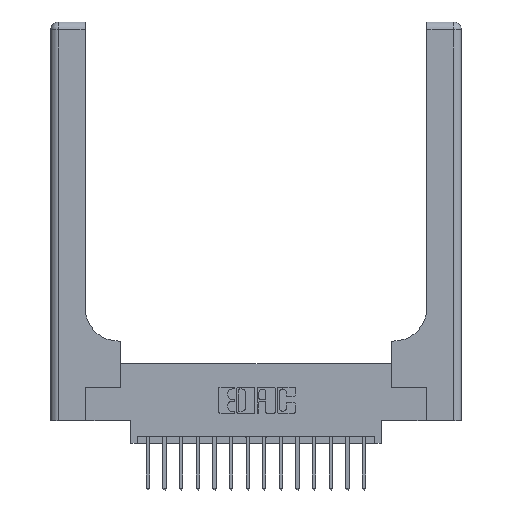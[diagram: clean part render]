
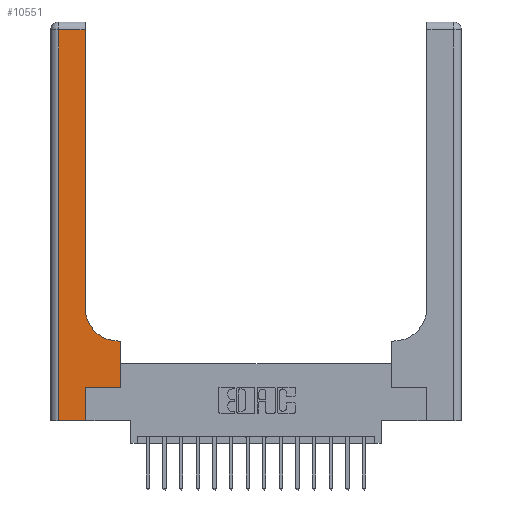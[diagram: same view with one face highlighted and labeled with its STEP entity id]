
A CAD part, top view. The second image highlights one B-rep face of the part: STEP entity #10551.
In plain terms, the highlighted planar face has unit normal (0, 0, 1).
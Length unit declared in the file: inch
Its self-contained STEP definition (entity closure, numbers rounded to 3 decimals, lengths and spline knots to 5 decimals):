
#180 = FACE_OUTER_BOUND ( 'NONE', #14261, .T. ) ;
#314 = LINE ( 'NONE', #7513, #13786 ) ;
#416 = DIRECTION ( 'NONE',  ( 0., 1., 0. ) ) ;
#673 = CARTESIAN_POINT ( 'NONE',  ( 0.26, 0.6, 0.37 ) ) ;
#781 = ORIENTED_EDGE ( 'NONE', *, *, #9626, .T. ) ;
#1243 = CARTESIAN_POINT ( 'NONE',  ( 0.265, 0., 0.37 ) ) ;
#1295 = VECTOR ( 'NONE', #16761, 39.37008 ) ;
#1492 = CARTESIAN_POINT ( 'NONE',  ( 0., 0., 0.37 ) ) ;
#2117 = LINE ( 'NONE', #7989, #9222 ) ;
#2170 = ORIENTED_EDGE ( 'NONE', *, *, #17997, .T. ) ;
#2189 = ORIENTED_EDGE ( 'NONE', *, *, #5326, .T. ) ;
#2384 = CARTESIAN_POINT ( 'NONE',  ( 0.26, 3., 0.37 ) ) ;
#2570 = LINE ( 'NONE', #18563, #8557 ) ;
#2741 = DIRECTION ( 'NONE',  ( 0., 1., 0. ) ) ;
#2985 = PLANE ( 'NONE',  #10521 ) ;
#3191 = VERTEX_POINT ( 'NONE', #1243 ) ;
#3690 = VERTEX_POINT ( 'NONE', #8817 ) ;
#3984 = ORIENTED_EDGE ( 'NONE', *, *, #6276, .T. ) ;
#4375 = VERTEX_POINT ( 'NONE', #17189 ) ;
#4446 = LINE ( 'NONE', #11925, #5252 ) ;
#4491 = CARTESIAN_POINT ( 'NONE',  ( 0.51, 0.6, 0.37 ) ) ;
#5035 = LINE ( 'NONE', #2384, #12600 ) ;
#5252 = VECTOR ( 'NONE', #5945, 39.37008 ) ;
#5265 = EDGE_CURVE ( 'NONE', #6155, #10819, #5832, .T. ) ;
#5299 = EDGE_CURVE ( 'NONE', #3690, #15250, #4446, .T. ) ;
#5326 = EDGE_CURVE ( 'NONE', #4375, #3191, #13040, .T. ) ;
#5688 = CARTESIAN_POINT ( 'NONE',  ( 0.26, 2.94, 0.37 ) ) ;
#5832 = CIRCLE ( 'NONE', #8265, 0.25 ) ;
#5945 = DIRECTION ( 'NONE',  ( 1., 0., 0. ) ) ;
#6155 = VERTEX_POINT ( 'NONE', #4491 ) ;
#6276 = EDGE_CURVE ( 'NONE', #15250, #17471, #2117, .T. ) ;
#6293 = CARTESIAN_POINT ( 'NONE',  ( 0.528, 0.6, 0.37 ) ) ;
#7513 = CARTESIAN_POINT ( 'NONE',  ( 0., 2.94, 0.37 ) ) ;
#7663 = EDGE_CURVE ( 'NONE', #12409, #4375, #16640, .T. ) ;
#7989 = CARTESIAN_POINT ( 'NONE',  ( 0.528, 0.25, 0.37 ) ) ;
#8265 = AXIS2_PLACEMENT_3D ( 'NONE', #15906, #8431, #14101 ) ;
#8411 = CARTESIAN_POINT ( 'NONE',  ( 0.528, 0.25, 0.37 ) ) ;
#8431 = DIRECTION ( 'NONE',  ( 0., 0., -1. ) ) ;
#8474 = EDGE_CURVE ( 'NONE', #10819, #14395, #5035, .T. ) ;
#8557 = VECTOR ( 'NONE', #2741, 39.37008 ) ;
#8711 = DIRECTION ( 'NONE',  ( 0., 0., -1. ) ) ;
#8817 = CARTESIAN_POINT ( 'NONE',  ( 0.265, 0.25, 0.37 ) ) ;
#9222 = VECTOR ( 'NONE', #416, 39.37008 ) ;
#9626 = EDGE_CURVE ( 'NONE', #14395, #12409, #314, .T. ) ;
#10186 = VECTOR ( 'NONE', #13886, 39.37008 ) ;
#10521 = AXIS2_PLACEMENT_3D ( 'NONE', #14467, #8711, #14655 ) ;
#10551 = ADVANCED_FACE ( 'NONE', ( #180 ), #2985, .F. ) ;
#10664 = ORIENTED_EDGE ( 'NONE', *, *, #5299, .T. ) ;
#10691 = ORIENTED_EDGE ( 'NONE', *, *, #17592, .T. ) ;
#10819 = VERTEX_POINT ( 'NONE', #12907 ) ;
#10843 = DIRECTION ( 'NONE',  ( 0., 1., 0. ) ) ;
#11101 = ORIENTED_EDGE ( 'NONE', *, *, #5265, .T. ) ;
#11925 = CARTESIAN_POINT ( 'NONE',  ( 0.265, 0.25, 0.37 ) ) ;
#12409 = VERTEX_POINT ( 'NONE', #15593 ) ;
#12600 = VECTOR ( 'NONE', #10843, 39.37008 ) ;
#12907 = CARTESIAN_POINT ( 'NONE',  ( 0.26, 0.85, 0.37 ) ) ;
#13040 = LINE ( 'NONE', #1492, #17947 ) ;
#13319 = DIRECTION ( 'NONE',  ( 1., 0., 0. ) ) ;
#13786 = VECTOR ( 'NONE', #16047, 39.37008 ) ;
#13886 = DIRECTION ( 'NONE',  ( 0., -1., 0. ) ) ;
#14063 = CARTESIAN_POINT ( 'NONE',  ( 0.06, 3., 0.37 ) ) ;
#14101 = DIRECTION ( 'NONE',  ( 1., 0., 0. ) ) ;
#14261 = EDGE_LOOP ( 'NONE', ( #18095, #781, #14748, #2189, #10691, #10664, #3984, #2170, #11101 ) ) ;
#14395 = VERTEX_POINT ( 'NONE', #5688 ) ;
#14467 = CARTESIAN_POINT ( 'NONE',  ( 0., 3., 0.37 ) ) ;
#14655 = DIRECTION ( 'NONE',  ( -1., 0., 0. ) ) ;
#14748 = ORIENTED_EDGE ( 'NONE', *, *, #7663, .T. ) ;
#15250 = VERTEX_POINT ( 'NONE', #8411 ) ;
#15593 = CARTESIAN_POINT ( 'NONE',  ( 0.06, 2.94, 0.37 ) ) ;
#15906 = CARTESIAN_POINT ( 'NONE',  ( 0.51, 0.85, 0.37 ) ) ;
#16047 = DIRECTION ( 'NONE',  ( -1., 0., 0. ) ) ;
#16595 = LINE ( 'NONE', #673, #1295 ) ;
#16640 = LINE ( 'NONE', #14063, #10186 ) ;
#16761 = DIRECTION ( 'NONE',  ( -1., 0., 0. ) ) ;
#17189 = CARTESIAN_POINT ( 'NONE',  ( 0.06, 0., 0.37 ) ) ;
#17471 = VERTEX_POINT ( 'NONE', #6293 ) ;
#17592 = EDGE_CURVE ( 'NONE', #3191, #3690, #2570, .T. ) ;
#17947 = VECTOR ( 'NONE', #13319, 39.37008 ) ;
#17997 = EDGE_CURVE ( 'NONE', #17471, #6155, #16595, .T. ) ;
#18095 = ORIENTED_EDGE ( 'NONE', *, *, #8474, .T. ) ;
#18563 = CARTESIAN_POINT ( 'NONE',  ( 0.265, 0., 0.37 ) ) ;
